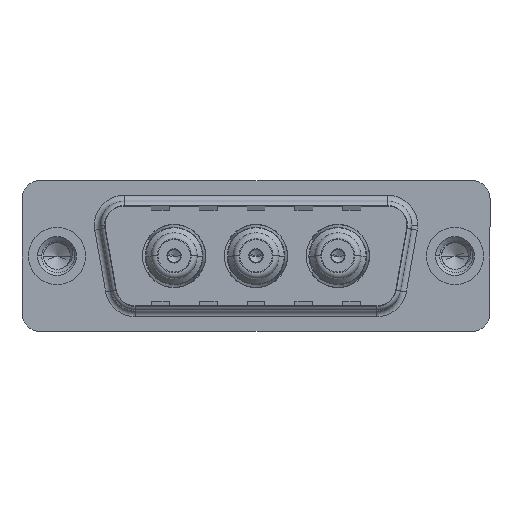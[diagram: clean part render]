
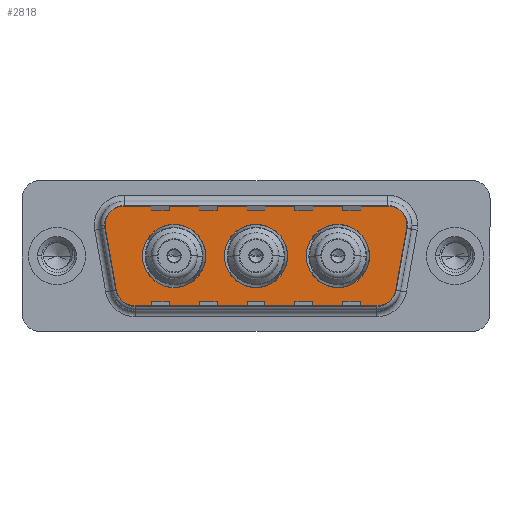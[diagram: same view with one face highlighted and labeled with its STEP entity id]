
A CAD part, top view. The second image highlights one B-rep face of the part: STEP entity #2818.
In plain terms, the highlighted planar face has unit normal (0, 0, 1).
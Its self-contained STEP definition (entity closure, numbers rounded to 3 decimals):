
#377 = CARTESIAN_POINT ( 'NONE',  ( 7.15, 0., 0. ) ) ;
#423 = DIRECTION ( 'NONE',  ( 1., 0., 0. ) ) ;
#438 = CIRCLE ( 'NONE', #8936, 2.65 ) ;
#495 = ORIENTED_EDGE ( 'NONE', *, *, #15472, .T. ) ;
#605 = VERTEX_POINT ( 'NONE', #8724 ) ;
#674 = DIRECTION ( 'NONE',  ( 1., 0., 0. ) ) ;
#675 = AXIS2_PLACEMENT_3D ( 'NONE', #823, #9694, #2171 ) ;
#715 = ORIENTED_EDGE ( 'NONE', *, *, #13229, .F. ) ;
#823 = CARTESIAN_POINT ( 'NONE',  ( 16.65, 0., 0. ) ) ;
#927 = DIRECTION ( 'NONE',  ( -1., 0., 0. ) ) ;
#1053 = FACE_BOUND ( 'NONE', #8321, .T. ) ;
#1055 = EDGE_CURVE ( 'NONE', #4933, #11044, #12548, .T. ) ;
#1224 = ORIENTED_EDGE ( 'NONE', *, *, #14287, .T. ) ;
#1244 = EDGE_LOOP ( 'NONE', ( #715, #12966 ) ) ;
#1282 = DIRECTION ( 'NONE',  ( 1., 0., 0. ) ) ;
#1338 = EDGE_CURVE ( 'NONE', #605, #4829, #9011, .T. ) ;
#1996 = VERTEX_POINT ( 'NONE', #7827 ) ;
#2022 = DIRECTION ( 'NONE',  ( 0., 0., 1. ) ) ;
#2122 = DIRECTION ( 'NONE',  ( 1., 0., 0. ) ) ;
#2143 = LINE ( 'NONE', #8219, #15510 ) ;
#2171 = DIRECTION ( 'NONE',  ( 1., 0., 0. ) ) ;
#2285 = CARTESIAN_POINT ( 'NONE',  ( 9.8, 0., 0. ) ) ;
#2591 = CARTESIAN_POINT ( 'NONE',  ( 6.434, -4.9, 0. ) ) ;
#2638 = CARTESIAN_POINT ( 'NONE',  ( 19.3, 0., 0. ) ) ;
#2656 = CARTESIAN_POINT ( 'NONE',  ( 14., 0., 0. ) ) ;
#2818 = ADVANCED_FACE ( 'NONE', ( #10740, #4556, #1053, #11164 ), #6682, .T. ) ;
#2956 = VERTEX_POINT ( 'NONE', #13662 ) ;
#2986 = EDGE_CURVE ( 'NONE', #1996, #2956, #5541, .T. ) ;
#3080 = VERTEX_POINT ( 'NONE', #15639 ) ;
#3154 = EDGE_CURVE ( 'NONE', #3080, #15719, #438, .T. ) ;
#3623 = DIRECTION ( 'NONE',  ( 1., 0., 0. ) ) ;
#3639 = CARTESIAN_POINT ( 'NONE',  ( 29.859, 2.553, 0. ) ) ;
#3870 = CARTESIAN_POINT ( 'NONE',  ( 4.464, -3.247, 0. ) ) ;
#3942 = CIRCLE ( 'NONE', #11647, 2. ) ;
#3951 = DIRECTION ( 'NONE',  ( 0., 0., 1. ) ) ;
#4001 = VECTOR ( 'NONE', #10234, 1000. ) ;
#4556 = FACE_BOUND ( 'NONE', #14711, .T. ) ;
#4612 = CARTESIAN_POINT ( 'NONE',  ( 29.889, 2.9, 0. ) ) ;
#4637 = DIRECTION ( 'NONE',  ( 0., 0., 1. ) ) ;
#4752 = ORIENTED_EDGE ( 'NONE', *, *, #11369, .T. ) ;
#4829 = VERTEX_POINT ( 'NONE', #12698 ) ;
#4933 = VERTEX_POINT ( 'NONE', #2656 ) ;
#4965 = AXIS2_PLACEMENT_3D ( 'NONE', #16368, #8867, #1282 ) ;
#5007 = CIRCLE ( 'NONE', #7187, 2. ) ;
#5116 = AXIS2_PLACEMENT_3D ( 'NONE', #14701, #3951, #14895 ) ;
#5134 = VECTOR ( 'NONE', #7907, 1000. ) ;
#5258 = CARTESIAN_POINT ( 'NONE',  ( 27.889, 2.9, 0. ) ) ;
#5324 = CIRCLE ( 'NONE', #675, 2.65 ) ;
#5441 = ORIENTED_EDGE ( 'NONE', *, *, #3154, .F. ) ;
#5541 = LINE ( 'NONE', #2591, #5134 ) ;
#6342 = CIRCLE ( 'NONE', #16114, 2.65 ) ;
#6507 = DIRECTION ( 'NONE',  ( -1., 0., 0. ) ) ;
#6509 = CARTESIAN_POINT ( 'NONE',  ( 3.441, 2.553, 0. ) ) ;
#6634 = CARTESIAN_POINT ( 'NONE',  ( 20.85, 0., 0. ) ) ;
#6682 = PLANE ( 'NONE',  #5116 ) ;
#7059 = DIRECTION ( 'NONE',  ( 0., 0., 1. ) ) ;
#7187 = AXIS2_PLACEMENT_3D ( 'NONE', #9539, #2022, #10802 ) ;
#7250 = ORIENTED_EDGE ( 'NONE', *, *, #1338, .T. ) ;
#7304 = LINE ( 'NONE', #6509, #4001 ) ;
#7383 = ORIENTED_EDGE ( 'NONE', *, *, #11810, .F. ) ;
#7411 = CARTESIAN_POINT ( 'NONE',  ( 5.411, 2.9, 0. ) ) ;
#7762 = AXIS2_PLACEMENT_3D ( 'NONE', #2285, #11077, #3623 ) ;
#7827 = CARTESIAN_POINT ( 'NONE',  ( 6.434, -4.9, 0. ) ) ;
#7907 = DIRECTION ( 'NONE',  ( 1., 0., 0. ) ) ;
#8051 = DIRECTION ( 'NONE',  ( 0., 0., 1. ) ) ;
#8188 = ORIENTED_EDGE ( 'NONE', *, *, #8757, .F. ) ;
#8219 = CARTESIAN_POINT ( 'NONE',  ( 5.411, 4.9, 0. ) ) ;
#8321 = EDGE_LOOP ( 'NONE', ( #5441, #8188 ) ) ;
#8447 = ORIENTED_EDGE ( 'NONE', *, *, #2986, .T. ) ;
#8463 = CARTESIAN_POINT ( 'NONE',  ( 27.889, 4.9, 0. ) ) ;
#8542 = DIRECTION ( 'NONE',  ( 0., 0., 1. ) ) ;
#8554 = VERTEX_POINT ( 'NONE', #14222 ) ;
#8724 = CARTESIAN_POINT ( 'NONE',  ( 5.411, 4.9, 0. ) ) ;
#8757 = EDGE_CURVE ( 'NONE', #15719, #3080, #9100, .T. ) ;
#8867 = DIRECTION ( 'NONE',  ( 0., 0., 1. ) ) ;
#8926 = EDGE_CURVE ( 'NONE', #13942, #11310, #10468, .T. ) ;
#8936 = AXIS2_PLACEMENT_3D ( 'NONE', #11744, #14798, #674 ) ;
#9011 = CIRCLE ( 'NONE', #14146, 2. ) ;
#9038 = DIRECTION ( 'NONE',  ( 1., 0., 0. ) ) ;
#9100 = CIRCLE ( 'NONE', #7762, 2.65 ) ;
#9458 = DIRECTION ( 'NONE',  ( -1., 0., 0. ) ) ;
#9539 = CARTESIAN_POINT ( 'NONE',  ( 26.866, -2.9, 0. ) ) ;
#9646 = LINE ( 'NONE', #3639, #16305 ) ;
#9694 = DIRECTION ( 'NONE',  ( 0., 0., 1. ) ) ;
#9711 = ORIENTED_EDGE ( 'NONE', *, *, #11738, .T. ) ;
#9884 = EDGE_CURVE ( 'NONE', #2956, #10231, #5007, .T. ) ;
#10004 = AXIS2_PLACEMENT_3D ( 'NONE', #5258, #13973, #6507 ) ;
#10050 = EDGE_CURVE ( 'NONE', #10231, #8554, #9646, .T. ) ;
#10231 = VERTEX_POINT ( 'NONE', #15258 ) ;
#10234 = DIRECTION ( 'NONE',  ( 0.174, -0.985, 0. ) ) ;
#10468 = CIRCLE ( 'NONE', #4965, 2.65 ) ;
#10740 = FACE_BOUND ( 'NONE', #1244, .T. ) ;
#10802 = DIRECTION ( 'NONE',  ( 1., 0., 0. ) ) ;
#10847 = EDGE_CURVE ( 'NONE', #4829, #15055, #7304, .T. ) ;
#11044 = VERTEX_POINT ( 'NONE', #2638 ) ;
#11060 = ORIENTED_EDGE ( 'NONE', *, *, #10847, .T. ) ;
#11077 = DIRECTION ( 'NONE',  ( 0., 0., 1. ) ) ;
#11095 = DIRECTION ( 'NONE',  ( 0.174, 0.985, 0. ) ) ;
#11164 = FACE_OUTER_BOUND ( 'NONE', #12426, .T. ) ;
#11310 = VERTEX_POINT ( 'NONE', #15630 ) ;
#11369 = EDGE_CURVE ( 'NONE', #16352, #605, #2143, .T. ) ;
#11524 = CARTESIAN_POINT ( 'NONE',  ( 16.65, 0., 0. ) ) ;
#11647 = AXIS2_PLACEMENT_3D ( 'NONE', #16051, #8542, #927 ) ;
#11738 = EDGE_CURVE ( 'NONE', #8554, #15877, #13734, .T. ) ;
#11744 = CARTESIAN_POINT ( 'NONE',  ( 9.8, 0., 0. ) ) ;
#11810 = EDGE_CURVE ( 'NONE', #11310, #13942, #6342, .T. ) ;
#12068 = AXIS2_PLACEMENT_3D ( 'NONE', #12082, #4637, #13331 ) ;
#12082 = CARTESIAN_POINT ( 'NONE',  ( 27.889, 2.9, 0. ) ) ;
#12426 = EDGE_LOOP ( 'NONE', ( #15675, #12640, #9711, #495, #4752, #7250, #11060, #1224, #8447 ) ) ;
#12548 = CIRCLE ( 'NONE', #14443, 2.65 ) ;
#12640 = ORIENTED_EDGE ( 'NONE', *, *, #10050, .T. ) ;
#12698 = CARTESIAN_POINT ( 'NONE',  ( 3.441, 2.553, 0. ) ) ;
#12966 = ORIENTED_EDGE ( 'NONE', *, *, #1055, .F. ) ;
#13071 = CIRCLE ( 'NONE', #12068, 2. ) ;
#13219 = DIRECTION ( 'NONE',  ( 0., 0., 1. ) ) ;
#13229 = EDGE_CURVE ( 'NONE', #11044, #4933, #5324, .T. ) ;
#13331 = DIRECTION ( 'NONE',  ( -1., 0., 0. ) ) ;
#13662 = CARTESIAN_POINT ( 'NONE',  ( 26.866, -4.9, 0. ) ) ;
#13734 = CIRCLE ( 'NONE', #10004, 2. ) ;
#13942 = VERTEX_POINT ( 'NONE', #6634 ) ;
#13973 = DIRECTION ( 'NONE',  ( 0., 0., 1. ) ) ;
#14146 = AXIS2_PLACEMENT_3D ( 'NONE', #7411, #7059, #9038 ) ;
#14222 = CARTESIAN_POINT ( 'NONE',  ( 29.859, 2.553, 0. ) ) ;
#14287 = EDGE_CURVE ( 'NONE', #15055, #1996, #3942, .T. ) ;
#14443 = AXIS2_PLACEMENT_3D ( 'NONE', #11524, #13219, #2122 ) ;
#14701 = CARTESIAN_POINT ( 'NONE',  ( 26.866, -2.9, 0. ) ) ;
#14711 = EDGE_LOOP ( 'NONE', ( #7383, #15171 ) ) ;
#14798 = DIRECTION ( 'NONE',  ( 0., 0., 1. ) ) ;
#14895 = DIRECTION ( 'NONE',  ( 1., 0., 0. ) ) ;
#15055 = VERTEX_POINT ( 'NONE', #3870 ) ;
#15171 = ORIENTED_EDGE ( 'NONE', *, *, #8926, .F. ) ;
#15258 = CARTESIAN_POINT ( 'NONE',  ( 28.836, -3.247, 0. ) ) ;
#15472 = EDGE_CURVE ( 'NONE', #15877, #16352, #13071, .T. ) ;
#15510 = VECTOR ( 'NONE', #9458, 1000. ) ;
#15562 = CARTESIAN_POINT ( 'NONE',  ( 23.5, 0., 0. ) ) ;
#15630 = CARTESIAN_POINT ( 'NONE',  ( 26.15, 0., 0. ) ) ;
#15639 = CARTESIAN_POINT ( 'NONE',  ( 12.45, 0., 0. ) ) ;
#15675 = ORIENTED_EDGE ( 'NONE', *, *, #9884, .T. ) ;
#15719 = VERTEX_POINT ( 'NONE', #377 ) ;
#15877 = VERTEX_POINT ( 'NONE', #4612 ) ;
#16051 = CARTESIAN_POINT ( 'NONE',  ( 6.434, -2.9, 0. ) ) ;
#16114 = AXIS2_PLACEMENT_3D ( 'NONE', #15562, #8051, #423 ) ;
#16305 = VECTOR ( 'NONE', #11095, 1000. ) ;
#16352 = VERTEX_POINT ( 'NONE', #8463 ) ;
#16368 = CARTESIAN_POINT ( 'NONE',  ( 23.5, 0., 0. ) ) ;
